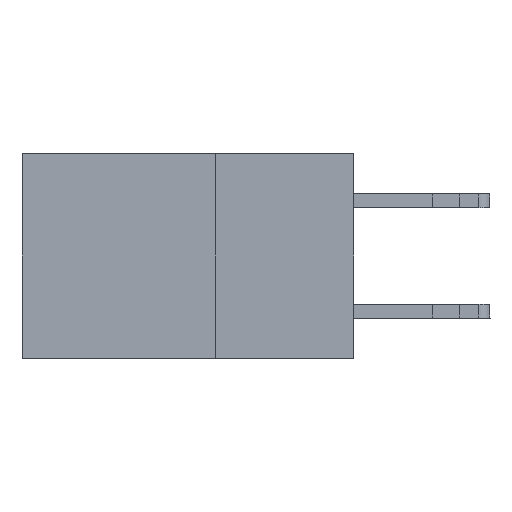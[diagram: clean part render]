
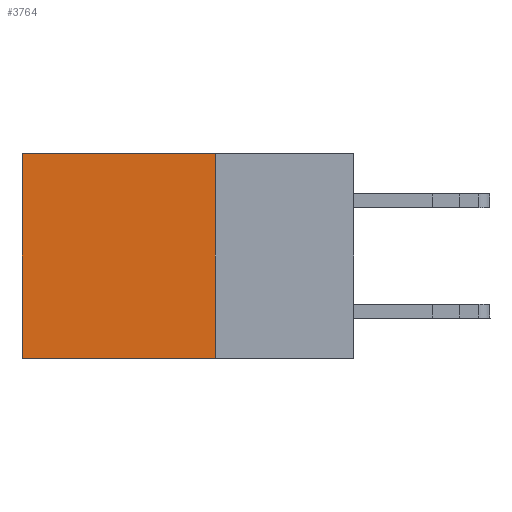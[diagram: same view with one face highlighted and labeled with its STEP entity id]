
A CAD part, left-side view. The second image highlights one B-rep face of the part: STEP entity #3764.
In plain terms, the highlighted planar face has unit normal (-1, 0, 0).
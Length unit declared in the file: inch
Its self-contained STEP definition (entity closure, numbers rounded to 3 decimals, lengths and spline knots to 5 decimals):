
#930 = CARTESIAN_POINT ( 'NONE',  ( 0.2875, 0.25, 0. ) ) ;
#958 = CARTESIAN_POINT ( 'NONE',  ( 0.2875, 0.6, -0.37 ) ) ;
#1575 = EDGE_CURVE ( 'NONE', #13345, #21612, #20828, .T. ) ;
#1900 = VERTEX_POINT ( 'NONE', #8988 ) ;
#2696 = VECTOR ( 'NONE', #3340, 39.37008 ) ;
#3264 = CARTESIAN_POINT ( 'NONE',  ( 0.2875, 0.25, -0.37 ) ) ;
#3267 = FACE_OUTER_BOUND ( 'NONE', #9449, .T. ) ;
#3340 = DIRECTION ( 'NONE',  ( 0., 0., -1. ) ) ;
#3764 = ADVANCED_FACE ( 'NONE', ( #3267 ), #14941, .F. ) ;
#3908 = CARTESIAN_POINT ( 'NONE',  ( 0.2875, 0.25, 0. ) ) ;
#4684 = DIRECTION ( 'NONE',  ( 0., 0., -1. ) ) ;
#5259 = ORIENTED_EDGE ( 'NONE', *, *, #20526, .F. ) ;
#6595 = LINE ( 'NONE', #23223, #2696 ) ;
#6625 = ORIENTED_EDGE ( 'NONE', *, *, #18135, .F. ) ;
#8036 = DIRECTION ( 'NONE',  ( 0., 1., 0. ) ) ;
#8988 = CARTESIAN_POINT ( 'NONE',  ( 0.2875, 0.25, -0.37 ) ) ;
#9052 = CARTESIAN_POINT ( 'NONE',  ( 0.2875, 0.6, 0. ) ) ;
#9449 = EDGE_LOOP ( 'NONE', ( #25102, #6625, #5259, #15448 ) ) ;
#9773 = VECTOR ( 'NONE', #20996, 39.37008 ) ;
#13283 = VECTOR ( 'NONE', #20934, 39.37008 ) ;
#13345 = VERTEX_POINT ( 'NONE', #19597 ) ;
#13560 = EDGE_CURVE ( 'NONE', #21612, #24330, #6595, .T. ) ;
#14923 = AXIS2_PLACEMENT_3D ( 'NONE', #3908, #24538, #4684 ) ;
#14941 = PLANE ( 'NONE',  #14923 ) ;
#15448 = ORIENTED_EDGE ( 'NONE', *, *, #1575, .T. ) ;
#18135 = EDGE_CURVE ( 'NONE', #1900, #24330, #20233, .T. ) ;
#19550 = LINE ( 'NONE', #930, #13283 ) ;
#19597 = CARTESIAN_POINT ( 'NONE',  ( 0.2875, 0.25, 0. ) ) ;
#20233 = LINE ( 'NONE', #3264, #9773 ) ;
#20526 = EDGE_CURVE ( 'NONE', #13345, #1900, #19550, .T. ) ;
#20828 = LINE ( 'NONE', #21561, #21192 ) ;
#20934 = DIRECTION ( 'NONE',  ( 0., 0., -1. ) ) ;
#20996 = DIRECTION ( 'NONE',  ( 0., 1., 0. ) ) ;
#21192 = VECTOR ( 'NONE', #8036, 39.37008 ) ;
#21561 = CARTESIAN_POINT ( 'NONE',  ( 0.2875, 0.25, 0. ) ) ;
#21612 = VERTEX_POINT ( 'NONE', #9052 ) ;
#23223 = CARTESIAN_POINT ( 'NONE',  ( 0.2875, 0.6, 0. ) ) ;
#24330 = VERTEX_POINT ( 'NONE', #958 ) ;
#24538 = DIRECTION ( 'NONE',  ( 1., 0., 0. ) ) ;
#25102 = ORIENTED_EDGE ( 'NONE', *, *, #13560, .T. ) ;
